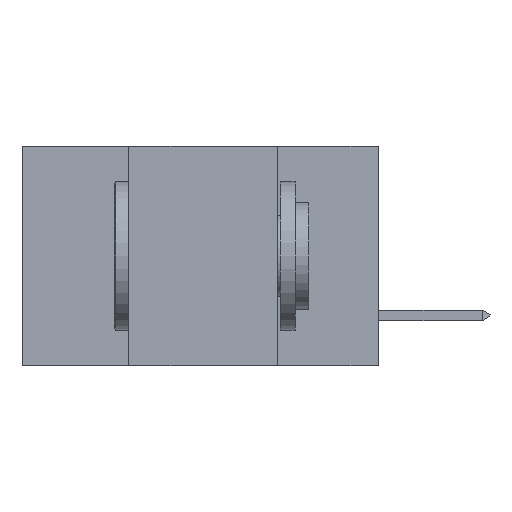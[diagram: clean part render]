
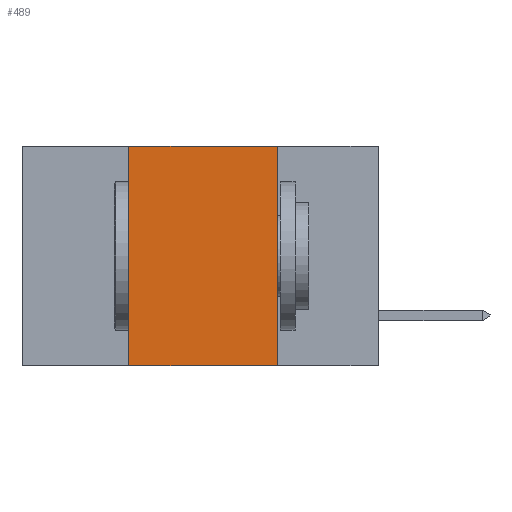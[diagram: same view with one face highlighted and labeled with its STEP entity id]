
A CAD part, left-side view. The second image highlights one B-rep face of the part: STEP entity #489.
In plain terms, the highlighted planar face has unit normal (-1, 0, 0).
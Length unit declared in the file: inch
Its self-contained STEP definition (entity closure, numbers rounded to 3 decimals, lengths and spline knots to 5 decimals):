
#489 = ADVANCED_FACE ( 'NONE', ( #12692 ), #1141, .F. ) ;
#828 = EDGE_CURVE ( 'NONE', #11915, #11086, #1396, .T. ) ;
#907 = LINE ( 'NONE', #5174, #12396 ) ;
#1125 = CARTESIAN_POINT ( 'NONE',  ( 0., 0.6, 0. ) ) ;
#1141 = PLANE ( 'NONE',  #7119 ) ;
#1396 = LINE ( 'NONE', #1125, #6677 ) ;
#1904 = LINE ( 'NONE', #10289, #5099 ) ;
#2383 = EDGE_CURVE ( 'NONE', #11086, #4424, #907, .T. ) ;
#2644 = CARTESIAN_POINT ( 'NONE',  ( 0., 0.17, -0.37 ) ) ;
#3328 = DIRECTION ( 'NONE',  ( 0., 0., -1. ) ) ;
#4424 = VERTEX_POINT ( 'NONE', #2644 ) ;
#4427 = DIRECTION ( 'NONE',  ( 1., 0., 0. ) ) ;
#4574 = ORIENTED_EDGE ( 'NONE', *, *, #828, .F. ) ;
#4866 = CARTESIAN_POINT ( 'NONE',  ( 0., 0.42, -0.37 ) ) ;
#4872 = EDGE_CURVE ( 'NONE', #9756, #11915, #10119, .T. ) ;
#5052 = DIRECTION ( 'NONE',  ( 0., -1., 0. ) ) ;
#5099 = VECTOR ( 'NONE', #5052, 39.37008 ) ;
#5174 = CARTESIAN_POINT ( 'NONE',  ( 0., 0.17, -0.37 ) ) ;
#5443 = VECTOR ( 'NONE', #10861, 39.37008 ) ;
#5776 = ORIENTED_EDGE ( 'NONE', *, *, #2383, .F. ) ;
#5840 = CARTESIAN_POINT ( 'NONE',  ( 0., 0.42, -0.37 ) ) ;
#6677 = VECTOR ( 'NONE', #8551, 39.37008 ) ;
#7119 = AXIS2_PLACEMENT_3D ( 'NONE', #12750, #4427, #3328 ) ;
#7236 = EDGE_LOOP ( 'NONE', ( #5776, #4574, #8514, #9112 ) ) ;
#8048 = CARTESIAN_POINT ( 'NONE',  ( 0., 0.17, 0. ) ) ;
#8514 = ORIENTED_EDGE ( 'NONE', *, *, #4872, .F. ) ;
#8551 = DIRECTION ( 'NONE',  ( 0., -1., 0. ) ) ;
#9112 = ORIENTED_EDGE ( 'NONE', *, *, #13271, .T. ) ;
#9181 = CARTESIAN_POINT ( 'NONE',  ( 0., 0.42, 0. ) ) ;
#9756 = VERTEX_POINT ( 'NONE', #4866 ) ;
#10119 = LINE ( 'NONE', #5840, #5443 ) ;
#10289 = CARTESIAN_POINT ( 'NONE',  ( 0., 0.6, -0.37 ) ) ;
#10477 = DIRECTION ( 'NONE',  ( 0., 0., -1. ) ) ;
#10861 = DIRECTION ( 'NONE',  ( 0., 0., 1. ) ) ;
#11086 = VERTEX_POINT ( 'NONE', #8048 ) ;
#11915 = VERTEX_POINT ( 'NONE', #9181 ) ;
#12396 = VECTOR ( 'NONE', #10477, 39.37008 ) ;
#12692 = FACE_OUTER_BOUND ( 'NONE', #7236, .T. ) ;
#12750 = CARTESIAN_POINT ( 'NONE',  ( 0., 0.6, 0. ) ) ;
#13271 = EDGE_CURVE ( 'NONE', #9756, #4424, #1904, .T. ) ;
